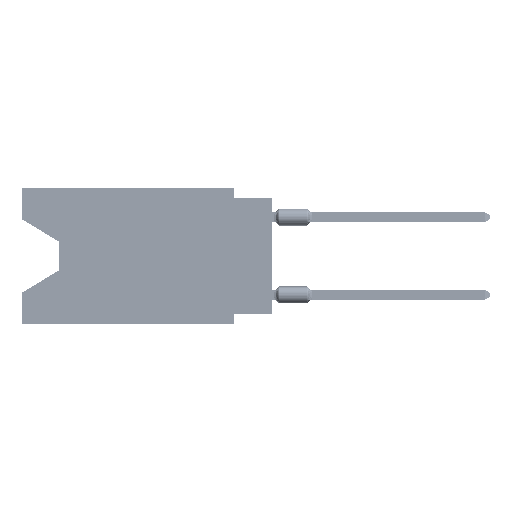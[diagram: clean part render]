
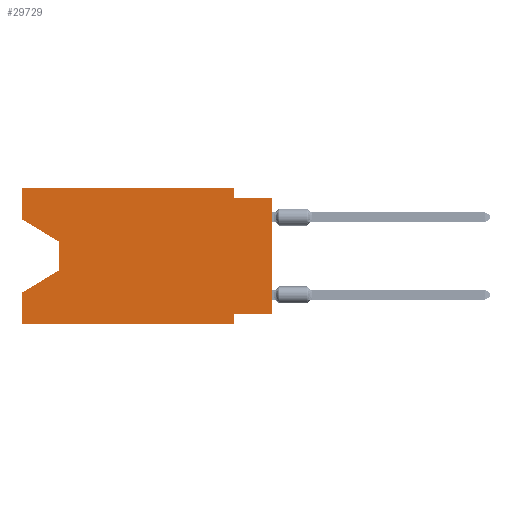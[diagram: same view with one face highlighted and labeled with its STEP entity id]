
A CAD part, left-side view. The second image highlights one B-rep face of the part: STEP entity #29729.
In plain terms, the highlighted planar face has unit normal (-1, 0, 0).
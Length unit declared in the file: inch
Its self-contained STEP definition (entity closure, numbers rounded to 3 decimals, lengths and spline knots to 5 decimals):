
#425 = VECTOR ( 'NONE', #103983, 39.37008 ) ;
#924 = CARTESIAN_POINT ( 'NONE',  ( 0., 0.1, -0.025 ) ) ;
#1130 = EDGE_CURVE ( 'NONE', #66980, #50940, #19226, .T. ) ;
#1652 = CARTESIAN_POINT ( 'NONE',  ( 0., 0.645, -0.35 ) ) ;
#1663 = VECTOR ( 'NONE', #35122, 39.37008 ) ;
#2892 = DIRECTION ( 'NONE',  ( 0., 0., 1. ) ) ;
#3892 = DIRECTION ( 'NONE',  ( 0., 0., -1. ) ) ;
#4700 = VERTEX_POINT ( 'NONE', #53295 ) ;
#5312 = VECTOR ( 'NONE', #105770, 39.37008 ) ;
#5488 = CARTESIAN_POINT ( 'NONE',  ( 0., 0.645, 0. ) ) ;
#6395 = LINE ( 'NONE', #81696, #27615 ) ;
#7746 = EDGE_CURVE ( 'NONE', #4700, #92633, #15754, .T. ) ;
#7941 = VERTEX_POINT ( 'NONE', #67025 ) ;
#7979 = ORIENTED_EDGE ( 'NONE', *, *, #60709, .T. ) ;
#8932 = CARTESIAN_POINT ( 'NONE',  ( 0., 0.55, -0.212 ) ) ;
#10581 = CARTESIAN_POINT ( 'NONE',  ( 0., 0.645, -0.35 ) ) ;
#11048 = ORIENTED_EDGE ( 'NONE', *, *, #93961, .T. ) ;
#11185 = DIRECTION ( 'NONE',  ( 0., -1., 0. ) ) ;
#12714 = ORIENTED_EDGE ( 'NONE', *, *, #70556, .T. ) ;
#13951 = VECTOR ( 'NONE', #45400, 39.37008 ) ;
#14024 = VECTOR ( 'NONE', #64623, 39.37008 ) ;
#14715 = EDGE_CURVE ( 'NONE', #107142, #58104, #21004, .T. ) ;
#15754 = LINE ( 'NONE', #41389, #60347 ) ;
#17384 = ORIENTED_EDGE ( 'NONE', *, *, #1130, .F. ) ;
#19226 = LINE ( 'NONE', #20315, #13951 ) ;
#20315 = CARTESIAN_POINT ( 'NONE',  ( 0., 0.645, 0. ) ) ;
#21004 = LINE ( 'NONE', #95235, #89635 ) ;
#23340 = CARTESIAN_POINT ( 'NONE',  ( 0., 0.1, 0. ) ) ;
#25566 = VECTOR ( 'NONE', #85660, 39.37008 ) ;
#26355 = VECTOR ( 'NONE', #50333, 39.37008 ) ;
#27615 = VECTOR ( 'NONE', #105737, 39.37008 ) ;
#27943 = VERTEX_POINT ( 'NONE', #8932 ) ;
#29729 = ADVANCED_FACE ( 'NONE', ( #96651 ), #36639, .F. ) ;
#29787 = DIRECTION ( 'NONE',  ( 0., -0.855, -0.519 ) ) ;
#30283 = CARTESIAN_POINT ( 'NONE',  ( 0., 0.55, -0.212 ) ) ;
#35122 = DIRECTION ( 'NONE',  ( 0., -1., 0. ) ) ;
#35296 = ORIENTED_EDGE ( 'NONE', *, *, #42832, .T. ) ;
#36639 = PLANE ( 'NONE',  #63216 ) ;
#38286 = CARTESIAN_POINT ( 'NONE',  ( 0., 0.55, -0.138 ) ) ;
#40774 = LINE ( 'NONE', #23340, #5312 ) ;
#41389 = CARTESIAN_POINT ( 'NONE',  ( 0., 0.1, -0.35 ) ) ;
#42447 = ORIENTED_EDGE ( 'NONE', *, *, #14715, .F. ) ;
#42832 = EDGE_CURVE ( 'NONE', #70224, #27943, #6395, .T. ) ;
#43637 = LINE ( 'NONE', #1652, #25566 ) ;
#45400 = DIRECTION ( 'NONE',  ( 0., 0., 1. ) ) ;
#45622 = CARTESIAN_POINT ( 'NONE',  ( 0., 0.645, -0.08025 ) ) ;
#45962 = LINE ( 'NONE', #54673, #63994 ) ;
#46370 = CARTESIAN_POINT ( 'NONE',  ( 0., 0.645, -0.08025 ) ) ;
#49599 = ORIENTED_EDGE ( 'NONE', *, *, #74753, .F. ) ;
#50333 = DIRECTION ( 'NONE',  ( 0., 1., 0. ) ) ;
#50940 = VERTEX_POINT ( 'NONE', #65287 ) ;
#52573 = CARTESIAN_POINT ( 'NONE',  ( 0., 0.645, 0. ) ) ;
#53295 = CARTESIAN_POINT ( 'NONE',  ( 0., 0.1, -0.325 ) ) ;
#53462 = VECTOR ( 'NONE', #29787, 39.37008 ) ;
#53493 = VERTEX_POINT ( 'NONE', #98748 ) ;
#54673 = CARTESIAN_POINT ( 'NONE',  ( 0., 0., 0. ) ) ;
#54870 = ORIENTED_EDGE ( 'NONE', *, *, #98621, .F. ) ;
#55204 = CARTESIAN_POINT ( 'NONE',  ( 0., 0., -0.025 ) ) ;
#58104 = VERTEX_POINT ( 'NONE', #55204 ) ;
#58454 = VERTEX_POINT ( 'NONE', #46370 ) ;
#58845 = CARTESIAN_POINT ( 'NONE',  ( 0., 0.645, 0. ) ) ;
#60347 = VECTOR ( 'NONE', #91043, 39.37008 ) ;
#60709 = EDGE_CURVE ( 'NONE', #27943, #50940, #105046, .T. ) ;
#62950 = ORIENTED_EDGE ( 'NONE', *, *, #73660, .F. ) ;
#62975 = CARTESIAN_POINT ( 'NONE',  ( 0., 0.645, 0. ) ) ;
#63216 = AXIS2_PLACEMENT_3D ( 'NONE', #5488, #104292, #3892 ) ;
#63966 = EDGE_CURVE ( 'NONE', #58454, #88435, #83939, .T. ) ;
#63994 = VECTOR ( 'NONE', #2892, 39.37008 ) ;
#64623 = DIRECTION ( 'NONE',  ( 0., 0.855, -0.519 ) ) ;
#65287 = CARTESIAN_POINT ( 'NONE',  ( 0., 0.645, -0.26975 ) ) ;
#66980 = VERTEX_POINT ( 'NONE', #10581 ) ;
#67025 = CARTESIAN_POINT ( 'NONE',  ( 0., 0.1, 0. ) ) ;
#70224 = VERTEX_POINT ( 'NONE', #38286 ) ;
#70556 = EDGE_CURVE ( 'NONE', #66980, #92633, #43637, .T. ) ;
#73660 = EDGE_CURVE ( 'NONE', #88435, #7941, #77704, .T. ) ;
#74195 = ORIENTED_EDGE ( 'NONE', *, *, #84337, .T. ) ;
#74366 = LINE ( 'NONE', #100538, #26355 ) ;
#74753 = EDGE_CURVE ( 'NONE', #7941, #107142, #40774, .T. ) ;
#75085 = ORIENTED_EDGE ( 'NONE', *, *, #63966, .F. ) ;
#77704 = LINE ( 'NONE', #52573, #1663 ) ;
#79136 = ORIENTED_EDGE ( 'NONE', *, *, #7746, .F. ) ;
#81696 = CARTESIAN_POINT ( 'NONE',  ( 0., 0.55, -0.138 ) ) ;
#83939 = LINE ( 'NONE', #58845, #425 ) ;
#84337 = EDGE_CURVE ( 'NONE', #53493, #58104, #45962, .T. ) ;
#85660 = DIRECTION ( 'NONE',  ( 0., -1., 0. ) ) ;
#88435 = VERTEX_POINT ( 'NONE', #62975 ) ;
#89635 = VECTOR ( 'NONE', #11185, 39.37008 ) ;
#91043 = DIRECTION ( 'NONE',  ( 0., 0., -1. ) ) ;
#92633 = VERTEX_POINT ( 'NONE', #93185 ) ;
#93185 = CARTESIAN_POINT ( 'NONE',  ( 0., 0.1, -0.35 ) ) ;
#93797 = EDGE_LOOP ( 'NONE', ( #11048, #35296, #7979, #17384, #12714, #79136, #54870, #74195, #42447, #49599, #62950, #75085 ) ) ;
#93961 = EDGE_CURVE ( 'NONE', #58454, #70224, #102927, .T. ) ;
#95235 = CARTESIAN_POINT ( 'NONE',  ( 0., 0., -0.025 ) ) ;
#96651 = FACE_OUTER_BOUND ( 'NONE', #93797, .T. ) ;
#98621 = EDGE_CURVE ( 'NONE', #53493, #4700, #74366, .T. ) ;
#98748 = CARTESIAN_POINT ( 'NONE',  ( 0., 0., -0.325 ) ) ;
#100538 = CARTESIAN_POINT ( 'NONE',  ( 0., 0., -0.325 ) ) ;
#102927 = LINE ( 'NONE', #45622, #53462 ) ;
#103983 = DIRECTION ( 'NONE',  ( 0., 0., 1. ) ) ;
#104292 = DIRECTION ( 'NONE',  ( 1., 0., 0. ) ) ;
#105046 = LINE ( 'NONE', #30283, #14024 ) ;
#105737 = DIRECTION ( 'NONE',  ( 0., 0., -1. ) ) ;
#105770 = DIRECTION ( 'NONE',  ( 0., 0., -1. ) ) ;
#107142 = VERTEX_POINT ( 'NONE', #924 ) ;
